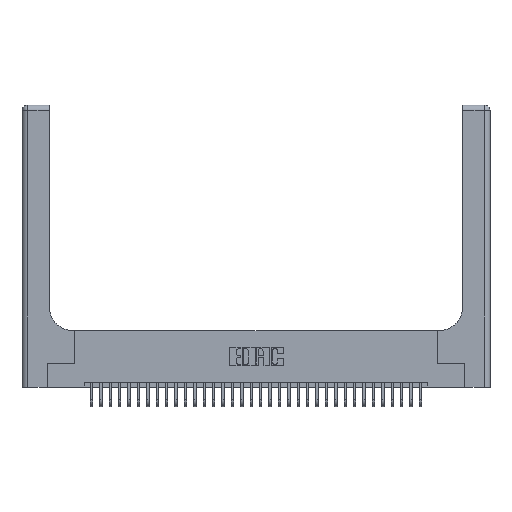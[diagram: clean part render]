
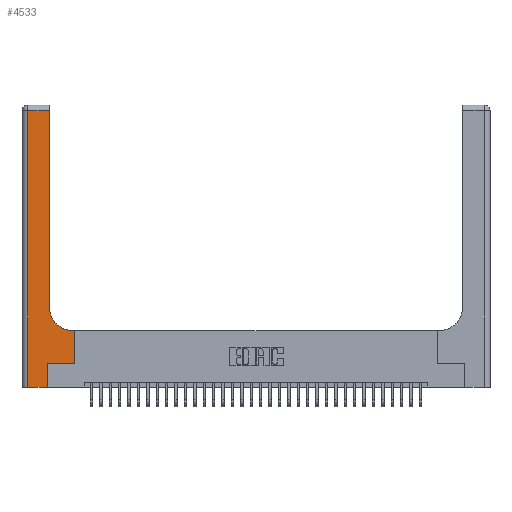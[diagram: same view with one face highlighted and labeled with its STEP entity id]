
A CAD part, top view. The second image highlights one B-rep face of the part: STEP entity #4533.
In plain terms, the highlighted planar face has unit normal (0, 0, 1).
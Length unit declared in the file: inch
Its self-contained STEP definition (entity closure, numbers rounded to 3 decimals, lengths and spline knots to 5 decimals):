
#10 = VECTOR ( 'NONE', #30217, 39.37008 ) ;
#719 = DIRECTION ( 'NONE',  ( -1., 0., 0. ) ) ;
#742 = CARTESIAN_POINT ( 'NONE',  ( 0., 0., 0.37 ) ) ;
#1918 = VECTOR ( 'NONE', #719, 39.37008 ) ;
#2465 = CARTESIAN_POINT ( 'NONE',  ( 0.5585, 0.25, 0.37 ) ) ;
#3304 = CARTESIAN_POINT ( 'NONE',  ( 0., 3., 0.37 ) ) ;
#3602 = AXIS2_PLACEMENT_3D ( 'NONE', #3304, #8851, #22914 ) ;
#3874 = VERTEX_POINT ( 'NONE', #28356 ) ;
#4197 = VERTEX_POINT ( 'NONE', #27574 ) ;
#4533 = ADVANCED_FACE ( 'NONE', ( #25808 ), #25455, .F. ) ;
#5039 = DIRECTION ( 'NONE',  ( -1., 0., 0. ) ) ;
#5256 = CARTESIAN_POINT ( 'NONE',  ( 0.269, 0., 0.37 ) ) ;
#5811 = EDGE_CURVE ( 'NONE', #18303, #11496, #21456, .T. ) ;
#6587 = ORIENTED_EDGE ( 'NONE', *, *, #12893, .T. ) ;
#8007 = AXIS2_PLACEMENT_3D ( 'NONE', #26098, #25974, #31763 ) ;
#8717 = VERTEX_POINT ( 'NONE', #34204 ) ;
#8851 = DIRECTION ( 'NONE',  ( 0., 0., -1. ) ) ;
#9092 = CARTESIAN_POINT ( 'NONE',  ( 0.269, 0.25, 0.37 ) ) ;
#9096 = CARTESIAN_POINT ( 'NONE',  ( 0., 2.94, 0.37 ) ) ;
#9161 = EDGE_CURVE ( 'NONE', #11496, #8717, #14772, .T. ) ;
#10245 = CARTESIAN_POINT ( 'NONE',  ( 0.06, 2.94, 0.37 ) ) ;
#10816 = EDGE_CURVE ( 'NONE', #34889, #4197, #32930, .T. ) ;
#11496 = VERTEX_POINT ( 'NONE', #12698 ) ;
#12594 = LINE ( 'NONE', #2465, #10 ) ;
#12698 = CARTESIAN_POINT ( 'NONE',  ( 0.269, 0.25, 0.37 ) ) ;
#12893 = EDGE_CURVE ( 'NONE', #23928, #32963, #34552, .T. ) ;
#13001 = CARTESIAN_POINT ( 'NONE',  ( 0.2915, 3., 0.37 ) ) ;
#13697 = VECTOR ( 'NONE', #32763, 39.37008 ) ;
#14479 = ORIENTED_EDGE ( 'NONE', *, *, #5811, .T. ) ;
#14772 = LINE ( 'NONE', #9092, #27416 ) ;
#16716 = ORIENTED_EDGE ( 'NONE', *, *, #26373, .T. ) ;
#16900 = LINE ( 'NONE', #742, #30436 ) ;
#17438 = DIRECTION ( 'NONE',  ( 1., 0., 0. ) ) ;
#18303 = VERTEX_POINT ( 'NONE', #5256 ) ;
#18598 = CARTESIAN_POINT ( 'NONE',  ( 0.269, 0., 0.37 ) ) ;
#18671 = ORIENTED_EDGE ( 'NONE', *, *, #31724, .T. ) ;
#21170 = EDGE_CURVE ( 'NONE', #31028, #23928, #30184, .T. ) ;
#21456 = LINE ( 'NONE', #18598, #24083 ) ;
#21851 = CARTESIAN_POINT ( 'NONE',  ( 0.2915, 0.6, 0.37 ) ) ;
#22764 = EDGE_LOOP ( 'NONE', ( #6587, #16716, #23635, #18671, #14479, #33223, #34722, #35503, #34344 ) ) ;
#22914 = DIRECTION ( 'NONE',  ( -1., 0., 0. ) ) ;
#23071 = CARTESIAN_POINT ( 'NONE',  ( 0.2915, 2.94, 0.37 ) ) ;
#23373 = CARTESIAN_POINT ( 'NONE',  ( 0.2915, 0.85, 0.37 ) ) ;
#23635 = ORIENTED_EDGE ( 'NONE', *, *, #10816, .T. ) ;
#23928 = VERTEX_POINT ( 'NONE', #23373 ) ;
#24083 = VECTOR ( 'NONE', #34623, 39.37008 ) ;
#25455 = PLANE ( 'NONE',  #3602 ) ;
#25808 = FACE_OUTER_BOUND ( 'NONE', #22764, .T. ) ;
#25974 = DIRECTION ( 'NONE',  ( 0., 0., -1. ) ) ;
#26098 = CARTESIAN_POINT ( 'NONE',  ( 0.5415, 0.85, 0.37 ) ) ;
#26373 = EDGE_CURVE ( 'NONE', #32963, #34889, #33153, .T. ) ;
#27038 = VECTOR ( 'NONE', #5039, 39.37008 ) ;
#27416 = VECTOR ( 'NONE', #17438, 39.37008 ) ;
#27574 = CARTESIAN_POINT ( 'NONE',  ( 0.06, 0., 0.37 ) ) ;
#28278 = DIRECTION ( 'NONE',  ( 1., 0., 0. ) ) ;
#28356 = CARTESIAN_POINT ( 'NONE',  ( 0.5585, 0.6, 0.37 ) ) ;
#28546 = VECTOR ( 'NONE', #31825, 39.37008 ) ;
#29062 = CARTESIAN_POINT ( 'NONE',  ( 0.06, 3., 0.37 ) ) ;
#30184 = CIRCLE ( 'NONE', #8007, 0.25 ) ;
#30217 = DIRECTION ( 'NONE',  ( 0., 1., 0. ) ) ;
#30436 = VECTOR ( 'NONE', #28278, 39.37008 ) ;
#30459 = EDGE_CURVE ( 'NONE', #3874, #31028, #30918, .T. ) ;
#30918 = LINE ( 'NONE', #21851, #27038 ) ;
#31028 = VERTEX_POINT ( 'NONE', #35513 ) ;
#31724 = EDGE_CURVE ( 'NONE', #4197, #18303, #16900, .T. ) ;
#31763 = DIRECTION ( 'NONE',  ( 1., 0., 0. ) ) ;
#31825 = DIRECTION ( 'NONE',  ( 0., -1., 0. ) ) ;
#32162 = EDGE_CURVE ( 'NONE', #8717, #3874, #12594, .T. ) ;
#32763 = DIRECTION ( 'NONE',  ( 0., 1., 0. ) ) ;
#32930 = LINE ( 'NONE', #29062, #28546 ) ;
#32963 = VERTEX_POINT ( 'NONE', #23071 ) ;
#33153 = LINE ( 'NONE', #9096, #1918 ) ;
#33223 = ORIENTED_EDGE ( 'NONE', *, *, #9161, .T. ) ;
#34204 = CARTESIAN_POINT ( 'NONE',  ( 0.5585, 0.25, 0.37 ) ) ;
#34344 = ORIENTED_EDGE ( 'NONE', *, *, #21170, .T. ) ;
#34552 = LINE ( 'NONE', #13001, #13697 ) ;
#34623 = DIRECTION ( 'NONE',  ( 0., 1., 0. ) ) ;
#34722 = ORIENTED_EDGE ( 'NONE', *, *, #32162, .T. ) ;
#34889 = VERTEX_POINT ( 'NONE', #10245 ) ;
#35503 = ORIENTED_EDGE ( 'NONE', *, *, #30459, .T. ) ;
#35513 = CARTESIAN_POINT ( 'NONE',  ( 0.5415, 0.6, 0.37 ) ) ;
